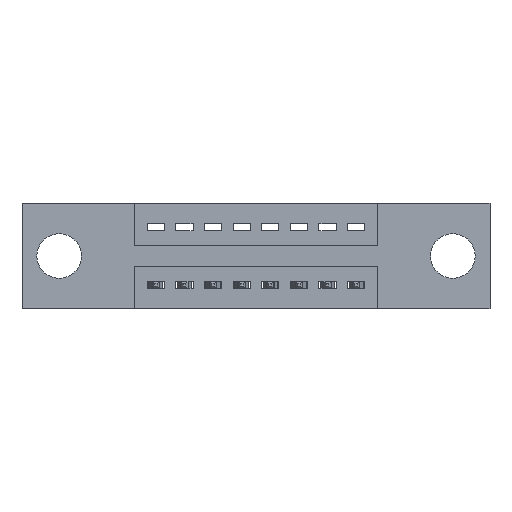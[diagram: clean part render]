
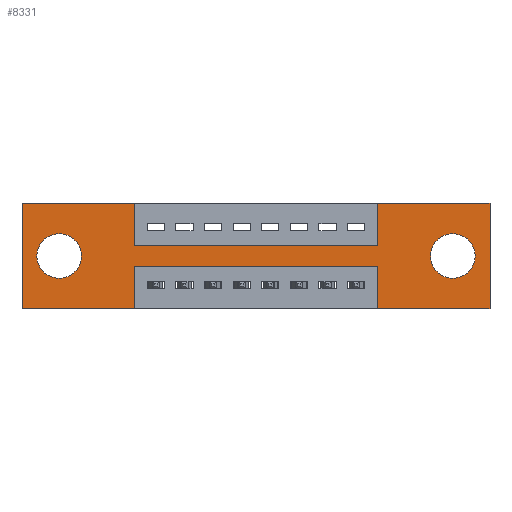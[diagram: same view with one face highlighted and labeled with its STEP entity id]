
A CAD part, front view. The second image highlights one B-rep face of the part: STEP entity #8331.
In plain terms, the highlighted planar face has unit normal (0, -1, 0).
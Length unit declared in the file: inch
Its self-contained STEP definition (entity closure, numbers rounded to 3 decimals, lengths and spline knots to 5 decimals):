
#58 = ORIENTED_EDGE ( 'NONE', *, *, #3178, .F. ) ;
#90 = PLANE ( 'NONE',  #8528 ) ;
#157 = LINE ( 'NONE', #8685, #4740 ) ;
#191 = VERTEX_POINT ( 'NONE', #9450 ) ;
#255 = FACE_BOUND ( 'NONE', #10001, .T. ) ;
#313 = VERTEX_POINT ( 'NONE', #3454 ) ;
#459 = EDGE_LOOP ( 'NONE', ( #6907, #4919 ) ) ;
#529 = DIRECTION ( 'NONE',  ( 0., 0., -1. ) ) ;
#634 = CARTESIAN_POINT ( 'NONE',  ( 0.3925, 0., -0.22 ) ) ;
#666 = CARTESIAN_POINT ( 'NONE',  ( 1.635, 0., 0. ) ) ;
#868 = DIRECTION ( 'NONE',  ( -1., 0., 0. ) ) ;
#913 = CARTESIAN_POINT ( 'NONE',  ( 0.13, 0., -0.185 ) ) ;
#1027 = CARTESIAN_POINT ( 'NONE',  ( 0.3925, 0., -0.22 ) ) ;
#1111 = CARTESIAN_POINT ( 'NONE',  ( 0.13, 0., -0.263 ) ) ;
#1170 = CARTESIAN_POINT ( 'NONE',  ( 1.505, 0., -0.185 ) ) ;
#1186 = VERTEX_POINT ( 'NONE', #2310 ) ;
#1269 = VECTOR ( 'NONE', #9966, 39.37008 ) ;
#1489 = VERTEX_POINT ( 'NONE', #1617 ) ;
#1576 = CARTESIAN_POINT ( 'NONE',  ( 0., 0., 0. ) ) ;
#1617 = CARTESIAN_POINT ( 'NONE',  ( 1.505, 0., -0.107 ) ) ;
#1618 = DIRECTION ( 'NONE',  ( 0., 0., 1. ) ) ;
#1770 = DIRECTION ( 'NONE',  ( 1., 0., 0. ) ) ;
#1890 = DIRECTION ( 'NONE',  ( 0., 0., 1. ) ) ;
#2023 = CARTESIAN_POINT ( 'NONE',  ( 1.2425, 0., -0.37 ) ) ;
#2026 = CARTESIAN_POINT ( 'NONE',  ( 1.505, 0., -0.185 ) ) ;
#2104 = DIRECTION ( 'NONE',  ( 0., -1., 0. ) ) ;
#2105 = CIRCLE ( 'NONE', #2658, 0.078 ) ;
#2131 = DIRECTION ( 'NONE',  ( 0., 0., -1. ) ) ;
#2310 = CARTESIAN_POINT ( 'NONE',  ( 0., 0., -0.37 ) ) ;
#2523 = CARTESIAN_POINT ( 'NONE',  ( 0., 0., 0. ) ) ;
#2658 = AXIS2_PLACEMENT_3D ( 'NONE', #913, #6894, #1890 ) ;
#2694 = DIRECTION ( 'NONE',  ( 0., 1., 0. ) ) ;
#2792 = FACE_BOUND ( 'NONE', #459, .T. ) ;
#2846 = ORIENTED_EDGE ( 'NONE', *, *, #4679, .F. ) ;
#2898 = DIRECTION ( 'NONE',  ( 0., 0., -1. ) ) ;
#3049 = VERTEX_POINT ( 'NONE', #1111 ) ;
#3172 = VERTEX_POINT ( 'NONE', #1576 ) ;
#3177 = VERTEX_POINT ( 'NONE', #1027 ) ;
#3178 = EDGE_CURVE ( 'NONE', #313, #3177, #6232, .T. ) ;
#3309 = VERTEX_POINT ( 'NONE', #4480 ) ;
#3366 = LINE ( 'NONE', #2023, #1269 ) ;
#3391 = EDGE_CURVE ( 'NONE', #9926, #313, #3366, .T. ) ;
#3454 = CARTESIAN_POINT ( 'NONE',  ( 1.2425, 0., -0.22 ) ) ;
#3611 = CARTESIAN_POINT ( 'NONE',  ( 0.3925, 0., 0. ) ) ;
#3744 = EDGE_CURVE ( 'NONE', #191, #3309, #4711, .T. ) ;
#3754 = CARTESIAN_POINT ( 'NONE',  ( 1.2425, 0., 0. ) ) ;
#3889 = CARTESIAN_POINT ( 'NONE',  ( 0.3925, 0., -0.15 ) ) ;
#4070 = VECTOR ( 'NONE', #9089, 39.37008 ) ;
#4080 = VECTOR ( 'NONE', #1618, 39.37008 ) ;
#4167 = VECTOR ( 'NONE', #1770, 39.37008 ) ;
#4297 = EDGE_CURVE ( 'NONE', #5355, #1186, #8153, .T. ) ;
#4321 = LINE ( 'NONE', #3889, #8302 ) ;
#4444 = VECTOR ( 'NONE', #529, 39.37008 ) ;
#4480 = CARTESIAN_POINT ( 'NONE',  ( 1.635, 0., -0.37 ) ) ;
#4606 = DIRECTION ( 'NONE',  ( 0., 0., 1. ) ) ;
#4678 = VERTEX_POINT ( 'NONE', #5898 ) ;
#4679 = EDGE_CURVE ( 'NONE', #3172, #5503, #8644, .T. ) ;
#4711 = LINE ( 'NONE', #666, #4444 ) ;
#4740 = VECTOR ( 'NONE', #8647, 39.37008 ) ;
#4918 = CARTESIAN_POINT ( 'NONE',  ( 0., 0., -0.37 ) ) ;
#4919 = ORIENTED_EDGE ( 'NONE', *, *, #9197, .T. ) ;
#4925 = LINE ( 'NONE', #3754, #8847 ) ;
#4965 = ORIENTED_EDGE ( 'NONE', *, *, #6754, .F. ) ;
#4967 = CARTESIAN_POINT ( 'NONE',  ( 0.3925, 0., 0. ) ) ;
#4984 = ORIENTED_EDGE ( 'NONE', *, *, #7474, .F. ) ;
#5018 = VECTOR ( 'NONE', #5547, 39.37008 ) ;
#5056 = CARTESIAN_POINT ( 'NONE',  ( 1.2425, 0., -0.15 ) ) ;
#5100 = ORIENTED_EDGE ( 'NONE', *, *, #6282, .F. ) ;
#5192 = ORIENTED_EDGE ( 'NONE', *, *, #9792, .F. ) ;
#5307 = CARTESIAN_POINT ( 'NONE',  ( 0.3925, 0., -0.15 ) ) ;
#5308 = AXIS2_PLACEMENT_3D ( 'NONE', #7601, #2694, #8400 ) ;
#5336 = ORIENTED_EDGE ( 'NONE', *, *, #10432, .F. ) ;
#5355 = VERTEX_POINT ( 'NONE', #5609 ) ;
#5364 = CARTESIAN_POINT ( 'NONE',  ( 0., 0., 0. ) ) ;
#5443 = ORIENTED_EDGE ( 'NONE', *, *, #3744, .F. ) ;
#5450 = CARTESIAN_POINT ( 'NONE',  ( 1.2425, 0., 0. ) ) ;
#5502 = CARTESIAN_POINT ( 'NONE',  ( 0., 0., -0.37 ) ) ;
#5503 = VERTEX_POINT ( 'NONE', #3611 ) ;
#5510 = CARTESIAN_POINT ( 'NONE',  ( 0.3925, 0., -0.37 ) ) ;
#5547 = DIRECTION ( 'NONE',  ( 0., 0., -1. ) ) ;
#5570 = ORIENTED_EDGE ( 'NONE', *, *, #6008, .F. ) ;
#5603 = VECTOR ( 'NONE', #868, 39.37008 ) ;
#5604 = ORIENTED_EDGE ( 'NONE', *, *, #4297, .F. ) ;
#5609 = CARTESIAN_POINT ( 'NONE',  ( 0.3925, 0., -0.37 ) ) ;
#5610 = LINE ( 'NONE', #4967, #9448 ) ;
#5613 = ORIENTED_EDGE ( 'NONE', *, *, #9020, .T. ) ;
#5760 = DIRECTION ( 'NONE',  ( 0., 0., -1. ) ) ;
#5783 = VERTEX_POINT ( 'NONE', #5307 ) ;
#5897 = VERTEX_POINT ( 'NONE', #5450 ) ;
#5898 = CARTESIAN_POINT ( 'NONE',  ( 0.13, 0., -0.107 ) ) ;
#5929 = ORIENTED_EDGE ( 'NONE', *, *, #3391, .F. ) ;
#5982 = EDGE_CURVE ( 'NONE', #3177, #5355, #9141, .T. ) ;
#6008 = EDGE_CURVE ( 'NONE', #3309, #9926, #157, .T. ) ;
#6186 = CARTESIAN_POINT ( 'NONE',  ( 1.505, 0., -0.263 ) ) ;
#6232 = LINE ( 'NONE', #634, #4070 ) ;
#6245 = LINE ( 'NONE', #2523, #4080 ) ;
#6282 = EDGE_CURVE ( 'NONE', #1186, #3172, #6245, .T. ) ;
#6533 = VECTOR ( 'NONE', #9211, 39.37008 ) ;
#6567 = AXIS2_PLACEMENT_3D ( 'NONE', #1170, #7090, #2131 ) ;
#6754 = EDGE_CURVE ( 'NONE', #5783, #10141, #4321, .T. ) ;
#6894 = DIRECTION ( 'NONE',  ( 0., 1., 0. ) ) ;
#6907 = ORIENTED_EDGE ( 'NONE', *, *, #10477, .T. ) ;
#7048 = EDGE_CURVE ( 'NONE', #3049, #4678, #7447, .T. ) ;
#7090 = DIRECTION ( 'NONE',  ( 0., 1., 0. ) ) ;
#7173 = FACE_OUTER_BOUND ( 'NONE', #7556, .T. ) ;
#7447 = CIRCLE ( 'NONE', #5308, 0.078 ) ;
#7474 = EDGE_CURVE ( 'NONE', #5503, #5783, #5610, .T. ) ;
#7556 = EDGE_LOOP ( 'NONE', ( #8274, #58, #5929, #5570, #5443, #5336, #5192, #4965, #4984, #2846, #5100, #5604 ) ) ;
#7601 = CARTESIAN_POINT ( 'NONE',  ( 0.13, 0., -0.185 ) ) ;
#7744 = AXIS2_PLACEMENT_3D ( 'NONE', #2026, #7782, #2898 ) ;
#7782 = DIRECTION ( 'NONE',  ( 0., 1., 0. ) ) ;
#7850 = DIRECTION ( 'NONE',  ( 0., 0., -1. ) ) ;
#7914 = DIRECTION ( 'NONE',  ( 1., 0., 0. ) ) ;
#7926 = CARTESIAN_POINT ( 'NONE',  ( 1.2425, 0., -0.37 ) ) ;
#8153 = LINE ( 'NONE', #4918, #5603 ) ;
#8207 = ORIENTED_EDGE ( 'NONE', *, *, #7048, .T. ) ;
#8274 = ORIENTED_EDGE ( 'NONE', *, *, #5982, .F. ) ;
#8302 = VECTOR ( 'NONE', #7914, 39.37008 ) ;
#8331 = ADVANCED_FACE ( 'NONE', ( #2792, #255, #7173 ), #90, .T. ) ;
#8400 = DIRECTION ( 'NONE',  ( 0., 0., 1. ) ) ;
#8528 = AXIS2_PLACEMENT_3D ( 'NONE', #5502, #2104, #7850 ) ;
#8644 = LINE ( 'NONE', #10265, #4167 ) ;
#8647 = DIRECTION ( 'NONE',  ( -1., 0., 0. ) ) ;
#8685 = CARTESIAN_POINT ( 'NONE',  ( 0., 0., -0.37 ) ) ;
#8847 = VECTOR ( 'NONE', #4606, 39.37008 ) ;
#9020 = EDGE_CURVE ( 'NONE', #4678, #3049, #2105, .T. ) ;
#9089 = DIRECTION ( 'NONE',  ( -1., 0., 0. ) ) ;
#9141 = LINE ( 'NONE', #5510, #5018 ) ;
#9197 = EDGE_CURVE ( 'NONE', #10454, #1489, #10573, .T. ) ;
#9211 = DIRECTION ( 'NONE',  ( 1., 0., 0. ) ) ;
#9448 = VECTOR ( 'NONE', #5760, 39.37008 ) ;
#9450 = CARTESIAN_POINT ( 'NONE',  ( 1.635, 0., 0. ) ) ;
#9792 = EDGE_CURVE ( 'NONE', #10141, #5897, #4925, .T. ) ;
#9926 = VERTEX_POINT ( 'NONE', #7926 ) ;
#9966 = DIRECTION ( 'NONE',  ( 0., 0., 1. ) ) ;
#10001 = EDGE_LOOP ( 'NONE', ( #5613, #8207 ) ) ;
#10037 = CIRCLE ( 'NONE', #7744, 0.078 ) ;
#10141 = VERTEX_POINT ( 'NONE', #5056 ) ;
#10265 = CARTESIAN_POINT ( 'NONE',  ( 0., 0., 0. ) ) ;
#10432 = EDGE_CURVE ( 'NONE', #5897, #191, #10451, .T. ) ;
#10451 = LINE ( 'NONE', #5364, #6533 ) ;
#10454 = VERTEX_POINT ( 'NONE', #6186 ) ;
#10477 = EDGE_CURVE ( 'NONE', #1489, #10454, #10037, .T. ) ;
#10573 = CIRCLE ( 'NONE', #6567, 0.078 ) ;
